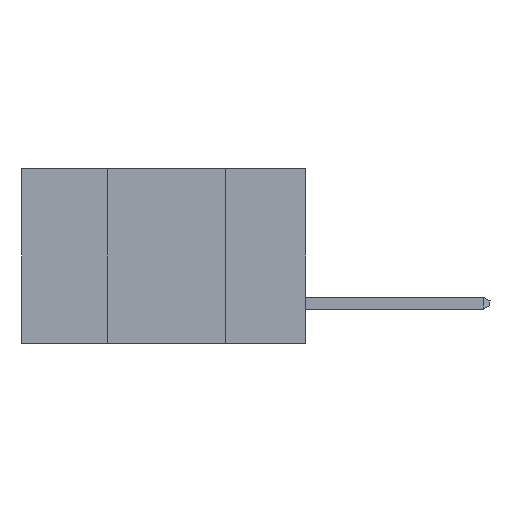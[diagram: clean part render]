
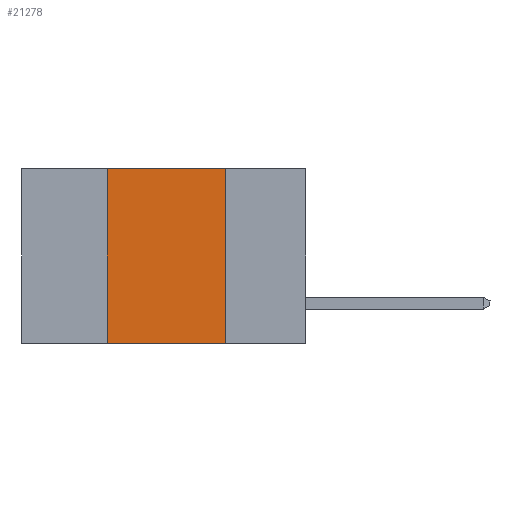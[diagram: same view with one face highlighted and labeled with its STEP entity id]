
A CAD part, left-side view. The second image highlights one B-rep face of the part: STEP entity #21278.
In plain terms, the highlighted planar face has unit normal (-1, 0, 0).
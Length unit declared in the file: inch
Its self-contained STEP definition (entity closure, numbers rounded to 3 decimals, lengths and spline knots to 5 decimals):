
#207 = EDGE_CURVE ( 'NONE', #8086, #9908, #18007, .T. ) ;
#470 = EDGE_CURVE ( 'NONE', #5725, #8086, #1536, .T. ) ;
#774 = CARTESIAN_POINT ( 'NONE',  ( 0., 0.17, -0.37 ) ) ;
#1043 = ORIENTED_EDGE ( 'NONE', *, *, #4122, .F. ) ;
#1536 = LINE ( 'NONE', #19716, #13406 ) ;
#2821 = LINE ( 'NONE', #17954, #5851 ) ;
#2978 = CARTESIAN_POINT ( 'NONE',  ( 0., 0.6, 0. ) ) ;
#3146 = DIRECTION ( 'NONE',  ( 0., -1., 0. ) ) ;
#3359 = DIRECTION ( 'NONE',  ( 0., 0., -1. ) ) ;
#4050 = LINE ( 'NONE', #774, #18918 ) ;
#4122 = EDGE_CURVE ( 'NONE', #9908, #19424, #4050, .T. ) ;
#4418 = AXIS2_PLACEMENT_3D ( 'NONE', #13167, #18494, #3359 ) ;
#5725 = VERTEX_POINT ( 'NONE', #9145 ) ;
#5851 = VECTOR ( 'NONE', #3146, 39.37008 ) ;
#8086 = VERTEX_POINT ( 'NONE', #12036 ) ;
#9145 = CARTESIAN_POINT ( 'NONE',  ( 0., 0.42, -0.37 ) ) ;
#9163 = DIRECTION ( 'NONE',  ( 0., 0., -1. ) ) ;
#9389 = DIRECTION ( 'NONE',  ( 0., 0., 1. ) ) ;
#9908 = VERTEX_POINT ( 'NONE', #13978 ) ;
#10965 = ORIENTED_EDGE ( 'NONE', *, *, #207, .F. ) ;
#11294 = EDGE_LOOP ( 'NONE', ( #1043, #10965, #21434, #11992 ) ) ;
#11992 = ORIENTED_EDGE ( 'NONE', *, *, #12184, .T. ) ;
#12036 = CARTESIAN_POINT ( 'NONE',  ( 0., 0.42, 0. ) ) ;
#12184 = EDGE_CURVE ( 'NONE', #5725, #19424, #2821, .T. ) ;
#13167 = CARTESIAN_POINT ( 'NONE',  ( 0., 0.6, 0. ) ) ;
#13406 = VECTOR ( 'NONE', #9389, 39.37008 ) ;
#13821 = CARTESIAN_POINT ( 'NONE',  ( 0., 0.17, -0.37 ) ) ;
#13978 = CARTESIAN_POINT ( 'NONE',  ( 0., 0.17, 0. ) ) ;
#14258 = VECTOR ( 'NONE', #17785, 39.37008 ) ;
#17785 = DIRECTION ( 'NONE',  ( 0., -1., 0. ) ) ;
#17954 = CARTESIAN_POINT ( 'NONE',  ( 0., 0.6, -0.37 ) ) ;
#18007 = LINE ( 'NONE', #2978, #14258 ) ;
#18068 = FACE_OUTER_BOUND ( 'NONE', #11294, .T. ) ;
#18281 = PLANE ( 'NONE',  #4418 ) ;
#18494 = DIRECTION ( 'NONE',  ( 1., 0., 0. ) ) ;
#18918 = VECTOR ( 'NONE', #9163, 39.37008 ) ;
#19424 = VERTEX_POINT ( 'NONE', #13821 ) ;
#19716 = CARTESIAN_POINT ( 'NONE',  ( 0., 0.42, -0.37 ) ) ;
#21278 = ADVANCED_FACE ( 'NONE', ( #18068 ), #18281, .F. ) ;
#21434 = ORIENTED_EDGE ( 'NONE', *, *, #470, .F. ) ;
